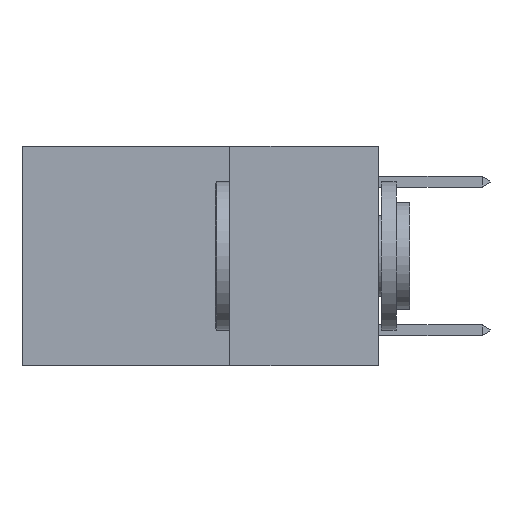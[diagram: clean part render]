
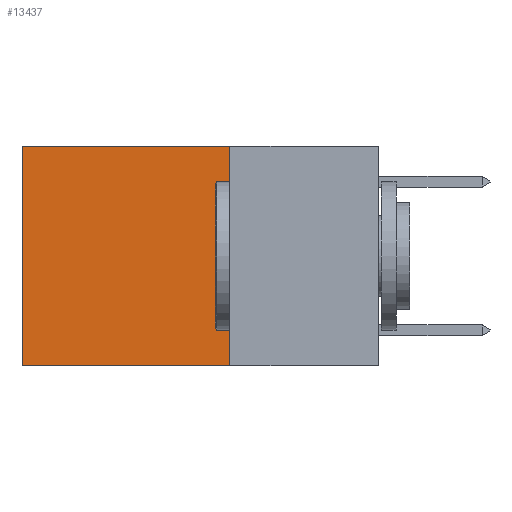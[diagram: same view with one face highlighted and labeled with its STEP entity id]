
A CAD part, left-side view. The second image highlights one B-rep face of the part: STEP entity #13437.
In plain terms, the highlighted planar face has unit normal (-1, 0, 0).
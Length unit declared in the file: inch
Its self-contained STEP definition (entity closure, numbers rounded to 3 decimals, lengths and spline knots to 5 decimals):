
#647 = LINE ( 'NONE', #11990, #4978 ) ;
#693 = VERTEX_POINT ( 'NONE', #6545 ) ;
#763 = VERTEX_POINT ( 'NONE', #11438 ) ;
#1646 = CARTESIAN_POINT ( 'NONE',  ( 0.2625, 0.25, 0. ) ) ;
#1853 = LINE ( 'NONE', #11127, #3501 ) ;
#2000 = EDGE_CURVE ( 'NONE', #3879, #763, #647, .T. ) ;
#2067 = DIRECTION ( 'NONE',  ( 0., 0., -1. ) ) ;
#3483 = CARTESIAN_POINT ( 'NONE',  ( 0.2625, 0.6, 0. ) ) ;
#3501 = VECTOR ( 'NONE', #2067, 39.37008 ) ;
#3879 = VERTEX_POINT ( 'NONE', #3483 ) ;
#3894 = CARTESIAN_POINT ( 'NONE',  ( 0.2625, 0.25, -0.37 ) ) ;
#4065 = DIRECTION ( 'NONE',  ( 0., 0., -1. ) ) ;
#4111 = ORIENTED_EDGE ( 'NONE', *, *, #14270, .F. ) ;
#4978 = VECTOR ( 'NONE', #4065, 39.37008 ) ;
#6029 = VERTEX_POINT ( 'NONE', #3894 ) ;
#6162 = DIRECTION ( 'NONE',  ( 0., 1., 0. ) ) ;
#6527 = FACE_OUTER_BOUND ( 'NONE', #9600, .T. ) ;
#6545 = CARTESIAN_POINT ( 'NONE',  ( 0.2625, 0.25, 0. ) ) ;
#7312 = VECTOR ( 'NONE', #6162, 39.37008 ) ;
#7548 = ORIENTED_EDGE ( 'NONE', *, *, #9341, .F. ) ;
#8755 = PLANE ( 'NONE',  #13034 ) ;
#9341 = EDGE_CURVE ( 'NONE', #693, #6029, #1853, .T. ) ;
#9600 = EDGE_LOOP ( 'NONE', ( #13143, #4111, #7548, #13388 ) ) ;
#9744 = DIRECTION ( 'NONE',  ( 0., 1., 0. ) ) ;
#10021 = DIRECTION ( 'NONE',  ( 1., 0., 0. ) ) ;
#10088 = CARTESIAN_POINT ( 'NONE',  ( 0.2625, 0.25, 0. ) ) ;
#10463 = EDGE_CURVE ( 'NONE', #693, #3879, #11813, .T. ) ;
#11127 = CARTESIAN_POINT ( 'NONE',  ( 0.2625, 0.25, 0. ) ) ;
#11438 = CARTESIAN_POINT ( 'NONE',  ( 0.2625, 0.6, -0.37 ) ) ;
#11813 = LINE ( 'NONE', #1646, #7312 ) ;
#11990 = CARTESIAN_POINT ( 'NONE',  ( 0.2625, 0.6, 0. ) ) ;
#13034 = AXIS2_PLACEMENT_3D ( 'NONE', #10088, #10021, #13413 ) ;
#13143 = ORIENTED_EDGE ( 'NONE', *, *, #2000, .T. ) ;
#13152 = LINE ( 'NONE', #14339, #13522 ) ;
#13388 = ORIENTED_EDGE ( 'NONE', *, *, #10463, .T. ) ;
#13413 = DIRECTION ( 'NONE',  ( 0., 0., -1. ) ) ;
#13437 = ADVANCED_FACE ( 'NONE', ( #6527 ), #8755, .F. ) ;
#13522 = VECTOR ( 'NONE', #9744, 39.37008 ) ;
#14270 = EDGE_CURVE ( 'NONE', #6029, #763, #13152, .T. ) ;
#14339 = CARTESIAN_POINT ( 'NONE',  ( 0.2625, 0.25, -0.37 ) ) ;
